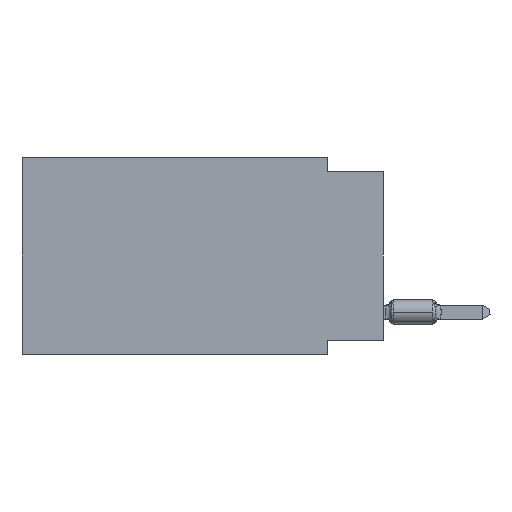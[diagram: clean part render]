
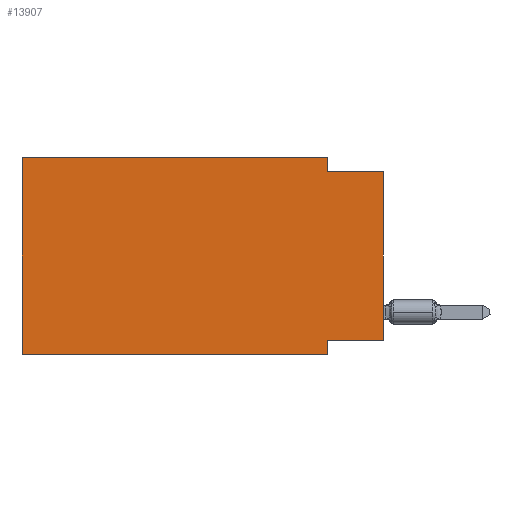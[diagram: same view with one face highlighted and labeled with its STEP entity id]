
A CAD part, left-side view. The second image highlights one B-rep face of the part: STEP entity #13907.
In plain terms, the highlighted planar face has unit normal (-1, 0, 0).
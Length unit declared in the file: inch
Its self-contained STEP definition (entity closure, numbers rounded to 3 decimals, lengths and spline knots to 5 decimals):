
#269 = VECTOR ( 'NONE', #2775, 39.37008 ) ;
#618 = LINE ( 'NONE', #15980, #47413 ) ;
#1758 = EDGE_CURVE ( 'NONE', #5479, #23960, #37745, .T. ) ;
#2228 = CARTESIAN_POINT ( 'NONE',  ( 0., 0.1, -0.025 ) ) ;
#2775 = DIRECTION ( 'NONE',  ( 0., -1., 0. ) ) ;
#4194 = CARTESIAN_POINT ( 'NONE',  ( 0., 0.1, -0.35 ) ) ;
#4535 = AXIS2_PLACEMENT_3D ( 'NONE', #8797, #28504, #39171 ) ;
#5479 = VERTEX_POINT ( 'NONE', #61705 ) ;
#7353 = DIRECTION ( 'NONE',  ( 0., 0., -1. ) ) ;
#8797 = CARTESIAN_POINT ( 'NONE',  ( 0., 0.645, 0. ) ) ;
#9084 = DIRECTION ( 'NONE',  ( 0., 1., 0. ) ) ;
#9339 = CARTESIAN_POINT ( 'NONE',  ( 0., 0.645, 0. ) ) ;
#9431 = EDGE_CURVE ( 'NONE', #54281, #12131, #61456, .T. ) ;
#10400 = CARTESIAN_POINT ( 'NONE',  ( 0., 0.645, -0.35 ) ) ;
#11424 = VECTOR ( 'NONE', #24971, 39.37008 ) ;
#12131 = VERTEX_POINT ( 'NONE', #51021 ) ;
#13907 = ADVANCED_FACE ( 'NONE', ( #53898 ), #38862, .F. ) ;
#15864 = EDGE_CURVE ( 'NONE', #38879, #12131, #27810, .T. ) ;
#15980 = CARTESIAN_POINT ( 'NONE',  ( 0., 0.645, 0. ) ) ;
#18271 = CARTESIAN_POINT ( 'NONE',  ( 0., 0.645, -0.35 ) ) ;
#18979 = VECTOR ( 'NONE', #9084, 39.37008 ) ;
#19497 = LINE ( 'NONE', #65604, #28188 ) ;
#21542 = ORIENTED_EDGE ( 'NONE', *, *, #40907, .F. ) ;
#22824 = CARTESIAN_POINT ( 'NONE',  ( 0., 0., -0.025 ) ) ;
#23391 = ORIENTED_EDGE ( 'NONE', *, *, #47531, .F. ) ;
#23960 = VERTEX_POINT ( 'NONE', #4194 ) ;
#24971 = DIRECTION ( 'NONE',  ( 0., 0., -1. ) ) ;
#25669 = ORIENTED_EDGE ( 'NONE', *, *, #40366, .T. ) ;
#27498 = VERTEX_POINT ( 'NONE', #43403 ) ;
#27810 = LINE ( 'NONE', #22824, #269 ) ;
#28188 = VECTOR ( 'NONE', #45182, 39.37008 ) ;
#28504 = DIRECTION ( 'NONE',  ( 1., 0., 0. ) ) ;
#29230 = EDGE_CURVE ( 'NONE', #43897, #27498, #618, .T. ) ;
#29386 = VECTOR ( 'NONE', #7353, 39.37008 ) ;
#31035 = DIRECTION ( 'NONE',  ( 0., 0., 1. ) ) ;
#33932 = EDGE_CURVE ( 'NONE', #27498, #38879, #55683, .T. ) ;
#35695 = VERTEX_POINT ( 'NONE', #10400 ) ;
#36892 = ORIENTED_EDGE ( 'NONE', *, *, #1758, .F. ) ;
#37745 = LINE ( 'NONE', #58132, #29386 ) ;
#38862 = PLANE ( 'NONE',  #4535 ) ;
#38879 = VERTEX_POINT ( 'NONE', #2228 ) ;
#39171 = DIRECTION ( 'NONE',  ( 0., 0., -1. ) ) ;
#40023 = EDGE_LOOP ( 'NONE', ( #55373, #52920, #50287, #46949, #21542, #25669, #36892, #23391 ) ) ;
#40366 = EDGE_CURVE ( 'NONE', #35695, #23960, #43300, .T. ) ;
#40741 = CARTESIAN_POINT ( 'NONE',  ( 0., 0., -0.325 ) ) ;
#40907 = EDGE_CURVE ( 'NONE', #35695, #43897, #19497, .T. ) ;
#43300 = LINE ( 'NONE', #18271, #47307 ) ;
#43403 = CARTESIAN_POINT ( 'NONE',  ( 0., 0.1, 0. ) ) ;
#43897 = VERTEX_POINT ( 'NONE', #9339 ) ;
#45182 = DIRECTION ( 'NONE',  ( 0., 0., 1. ) ) ;
#45466 = LINE ( 'NONE', #54835, #18979 ) ;
#46949 = ORIENTED_EDGE ( 'NONE', *, *, #29230, .F. ) ;
#47307 = VECTOR ( 'NONE', #63052, 39.37008 ) ;
#47413 = VECTOR ( 'NONE', #57389, 39.37008 ) ;
#47531 = EDGE_CURVE ( 'NONE', #54281, #5479, #45466, .T. ) ;
#50287 = ORIENTED_EDGE ( 'NONE', *, *, #33932, .F. ) ;
#51021 = CARTESIAN_POINT ( 'NONE',  ( 0., 0., -0.025 ) ) ;
#52067 = CARTESIAN_POINT ( 'NONE',  ( 0., 0., 0. ) ) ;
#52920 = ORIENTED_EDGE ( 'NONE', *, *, #15864, .F. ) ;
#53898 = FACE_OUTER_BOUND ( 'NONE', #40023, .T. ) ;
#54136 = VECTOR ( 'NONE', #31035, 39.37008 ) ;
#54281 = VERTEX_POINT ( 'NONE', #40741 ) ;
#54835 = CARTESIAN_POINT ( 'NONE',  ( 0., 0., -0.325 ) ) ;
#55373 = ORIENTED_EDGE ( 'NONE', *, *, #9431, .T. ) ;
#55683 = LINE ( 'NONE', #60703, #11424 ) ;
#57389 = DIRECTION ( 'NONE',  ( 0., -1., 0. ) ) ;
#58132 = CARTESIAN_POINT ( 'NONE',  ( 0., 0.1, -0.35 ) ) ;
#60703 = CARTESIAN_POINT ( 'NONE',  ( 0., 0.1, 0. ) ) ;
#61456 = LINE ( 'NONE', #52067, #54136 ) ;
#61705 = CARTESIAN_POINT ( 'NONE',  ( 0., 0.1, -0.325 ) ) ;
#63052 = DIRECTION ( 'NONE',  ( 0., -1., 0. ) ) ;
#65604 = CARTESIAN_POINT ( 'NONE',  ( 0., 0.645, 0. ) ) ;
